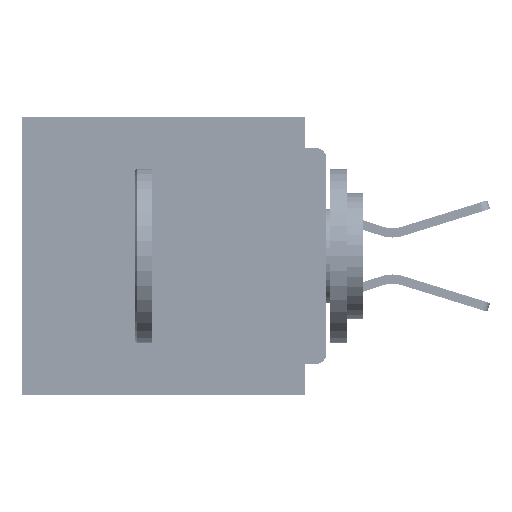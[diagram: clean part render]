
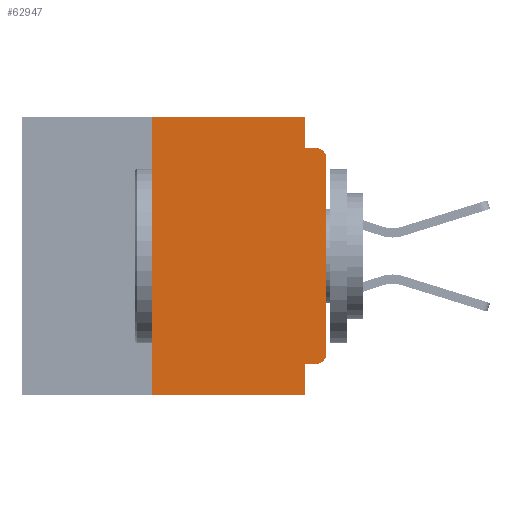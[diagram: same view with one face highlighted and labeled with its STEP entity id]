
A CAD part, left-side view. The second image highlights one B-rep face of the part: STEP entity #62947.
In plain terms, the highlighted planar face has unit normal (-1, 0, 0).
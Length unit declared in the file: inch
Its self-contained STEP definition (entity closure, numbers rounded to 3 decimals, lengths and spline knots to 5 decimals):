
#735 = DIRECTION ( 'NONE',  ( 0., 1., 0. ) ) ;
#2766 = CARTESIAN_POINT ( 'NONE',  ( 0., 0.437, 0. ) ) ;
#3372 = CARTESIAN_POINT ( 'NONE',  ( 0., 0., -0.045 ) ) ;
#4878 = CARTESIAN_POINT ( 'NONE',  ( 0., 0.015, -0.06 ) ) ;
#5505 = CIRCLE ( 'NONE', #52742, 0.015 ) ;
#6216 = CARTESIAN_POINT ( 'NONE',  ( 0., 0., 0. ) ) ;
#6428 = DIRECTION ( 'NONE',  ( 0., 0., 1. ) ) ;
#7182 = VERTEX_POINT ( 'NONE', #28917 ) ;
#7869 = DIRECTION ( 'NONE',  ( 0., 0., -1. ) ) ;
#8476 = ORIENTED_EDGE ( 'NONE', *, *, #42804, .F. ) ;
#8487 = DIRECTION ( 'NONE',  ( 0., -1., 0. ) ) ;
#9965 = DIRECTION ( 'NONE',  ( 0., 0., -1. ) ) ;
#10251 = EDGE_LOOP ( 'NONE', ( #42656, #64039, #8476, #23162, #44833, #29166, #64053, #44643, #26596, #31629 ) ) ;
#13455 = CARTESIAN_POINT ( 'NONE',  ( 0., 0.031, 0. ) ) ;
#13598 = VERTEX_POINT ( 'NONE', #15360 ) ;
#13969 = VECTOR ( 'NONE', #6428, 39.37008 ) ;
#14205 = VECTOR ( 'NONE', #8487, 39.37008 ) ;
#14369 = LINE ( 'NONE', #33236, #26101 ) ;
#14631 = CARTESIAN_POINT ( 'NONE',  ( 0., 0., -0.34 ) ) ;
#15360 = CARTESIAN_POINT ( 'NONE',  ( 0., 0.031, -0.4 ) ) ;
#16350 = LINE ( 'NONE', #20807, #28065 ) ;
#19124 = VERTEX_POINT ( 'NONE', #14631 ) ;
#20250 = EDGE_CURVE ( 'NONE', #23359, #19124, #5505, .T. ) ;
#20662 = EDGE_CURVE ( 'NONE', #39659, #62373, #44778, .T. ) ;
#20807 = CARTESIAN_POINT ( 'NONE',  ( 0., 0., -0.355 ) ) ;
#23162 = ORIENTED_EDGE ( 'NONE', *, *, #62017, .F. ) ;
#23359 = VERTEX_POINT ( 'NONE', #23664 ) ;
#23664 = CARTESIAN_POINT ( 'NONE',  ( 0., 0.015, -0.355 ) ) ;
#23897 = VERTEX_POINT ( 'NONE', #37775 ) ;
#24225 = LINE ( 'NONE', #29983, #34360 ) ;
#26101 = VECTOR ( 'NONE', #38264, 39.37008 ) ;
#26596 = ORIENTED_EDGE ( 'NONE', *, *, #60196, .F. ) ;
#27909 = CARTESIAN_POINT ( 'NONE',  ( 0., 0.25, 0. ) ) ;
#28065 = VECTOR ( 'NONE', #735, 39.37008 ) ;
#28917 = CARTESIAN_POINT ( 'NONE',  ( 0., 0.25, -0.4 ) ) ;
#29136 = CARTESIAN_POINT ( 'NONE',  ( 0., 0.015, -0.34 ) ) ;
#29166 = ORIENTED_EDGE ( 'NONE', *, *, #60077, .F. ) ;
#29983 = CARTESIAN_POINT ( 'NONE',  ( 0., 0.25, -0.4 ) ) ;
#31465 = VECTOR ( 'NONE', #47456, 39.37008 ) ;
#31629 = ORIENTED_EDGE ( 'NONE', *, *, #20250, .T. ) ;
#33236 = CARTESIAN_POINT ( 'NONE',  ( 0., 0.031, -0.4 ) ) ;
#33961 = VERTEX_POINT ( 'NONE', #54315 ) ;
#34153 = DIRECTION ( 'NONE',  ( 0., 0., -1. ) ) ;
#34360 = VECTOR ( 'NONE', #59930, 39.37008 ) ;
#36766 = CARTESIAN_POINT ( 'NONE',  ( 0., 0., -0.06 ) ) ;
#36947 = CIRCLE ( 'NONE', #43805, 0.015 ) ;
#37373 = CARTESIAN_POINT ( 'NONE',  ( 0., 0.437, 0. ) ) ;
#37775 = CARTESIAN_POINT ( 'NONE',  ( 0., 0.031, -0.045 ) ) ;
#37864 = DIRECTION ( 'NONE',  ( 1., 0., 0. ) ) ;
#37932 = EDGE_CURVE ( 'NONE', #19124, #62836, #40569, .T. ) ;
#38264 = DIRECTION ( 'NONE',  ( 0., 0., -1. ) ) ;
#39659 = VERTEX_POINT ( 'NONE', #27909 ) ;
#39933 = DIRECTION ( 'NONE',  ( -1., 0., 0. ) ) ;
#40569 = LINE ( 'NONE', #6216, #13969 ) ;
#41135 = VECTOR ( 'NONE', #55034, 39.37008 ) ;
#42656 = ORIENTED_EDGE ( 'NONE', *, *, #37932, .T. ) ;
#42687 = CARTESIAN_POINT ( 'NONE',  ( 0., 0.437, -0.4 ) ) ;
#42804 = EDGE_CURVE ( 'NONE', #23897, #33961, #54102, .T. ) ;
#43805 = AXIS2_PLACEMENT_3D ( 'NONE', #4878, #39933, #9965 ) ;
#44499 = CARTESIAN_POINT ( 'NONE',  ( 0., 0.031, -0.355 ) ) ;
#44643 = ORIENTED_EDGE ( 'NONE', *, *, #58334, .F. ) ;
#44778 = LINE ( 'NONE', #37373, #31465 ) ;
#44833 = ORIENTED_EDGE ( 'NONE', *, *, #20662, .F. ) ;
#46686 = EDGE_CURVE ( 'NONE', #62836, #33961, #36947, .T. ) ;
#47456 = DIRECTION ( 'NONE',  ( 0., -1., 0. ) ) ;
#47707 = DIRECTION ( 'NONE',  ( 0., -1., 0. ) ) ;
#47803 = VECTOR ( 'NONE', #47707, 39.37008 ) ;
#49635 = FACE_OUTER_BOUND ( 'NONE', #10251, .T. ) ;
#50005 = CARTESIAN_POINT ( 'NONE',  ( 0., 0.031, 0. ) ) ;
#52742 = AXIS2_PLACEMENT_3D ( 'NONE', #29136, #64114, #34153 ) ;
#52762 = PLANE ( 'NONE',  #61010 ) ;
#52894 = LINE ( 'NONE', #50005, #41135 ) ;
#54102 = LINE ( 'NONE', #3372, #14205 ) ;
#54315 = CARTESIAN_POINT ( 'NONE',  ( 0., 0.015, -0.045 ) ) ;
#55034 = DIRECTION ( 'NONE',  ( 0., 0., -1. ) ) ;
#57973 = LINE ( 'NONE', #42687, #47803 ) ;
#58334 = EDGE_CURVE ( 'NONE', #59529, #13598, #14369, .T. ) ;
#59529 = VERTEX_POINT ( 'NONE', #44499 ) ;
#59930 = DIRECTION ( 'NONE',  ( 0., 0., 1. ) ) ;
#60077 = EDGE_CURVE ( 'NONE', #7182, #39659, #24225, .T. ) ;
#60196 = EDGE_CURVE ( 'NONE', #23359, #59529, #16350, .T. ) ;
#61010 = AXIS2_PLACEMENT_3D ( 'NONE', #2766, #37864, #7869 ) ;
#62017 = EDGE_CURVE ( 'NONE', #62373, #23897, #52894, .T. ) ;
#62373 = VERTEX_POINT ( 'NONE', #13455 ) ;
#62836 = VERTEX_POINT ( 'NONE', #36766 ) ;
#62947 = ADVANCED_FACE ( 'NONE', ( #49635 ), #52762, .F. ) ;
#64039 = ORIENTED_EDGE ( 'NONE', *, *, #46686, .T. ) ;
#64053 = ORIENTED_EDGE ( 'NONE', *, *, #64841, .T. ) ;
#64114 = DIRECTION ( 'NONE',  ( -1., 0., 0. ) ) ;
#64841 = EDGE_CURVE ( 'NONE', #7182, #13598, #57973, .T. ) ;
